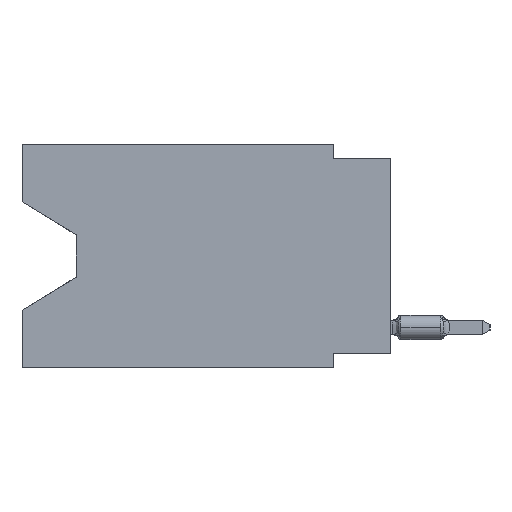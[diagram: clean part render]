
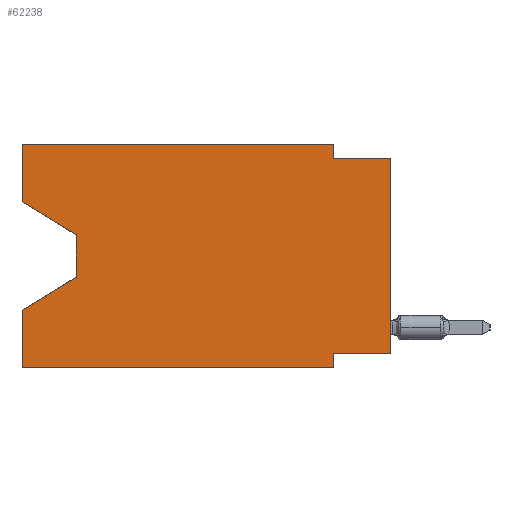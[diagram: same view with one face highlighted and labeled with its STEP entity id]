
A CAD part, left-side view. The second image highlights one B-rep face of the part: STEP entity #62238.
In plain terms, the highlighted planar face has unit normal (-1, 0, 0).
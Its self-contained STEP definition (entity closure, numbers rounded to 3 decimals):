
#249 = DIRECTION ( 'NONE',  ( 0., -0.855, -0.519 ) ) ;
#946 = ORIENTED_EDGE ( 'NONE', *, *, #59350, .F. ) ;
#1407 = PLANE ( 'NONE',  #7633 ) ;
#1590 = LINE ( 'NONE', #39635, #60868 ) ;
#2728 = VERTEX_POINT ( 'NONE', #63224 ) ;
#3511 = DIRECTION ( 'NONE',  ( 0., 0., 1. ) ) ;
#5503 = LINE ( 'NONE', #48896, #59118 ) ;
#5581 = EDGE_CURVE ( 'NONE', #42750, #20444, #65869, .T. ) ;
#6295 = CARTESIAN_POINT ( 'NONE',  ( 0., 16.383, -2.546 ) ) ;
#7633 = AXIS2_PLACEMENT_3D ( 'NONE', #13825, #45502, #29827 ) ;
#7803 = CARTESIAN_POINT ( 'NONE',  ( 0., 16.383, 0. ) ) ;
#7955 = CARTESIAN_POINT ( 'NONE',  ( 0., 16.383, -9.906 ) ) ;
#8317 = EDGE_CURVE ( 'NONE', #41188, #2728, #55021, .T. ) ;
#9799 = EDGE_LOOP ( 'NONE', ( #11325, #43804, #39291, #16638, #15266, #60975, #36947, #10320, #946, #68223, #22908, #34133 ) ) ;
#10320 = ORIENTED_EDGE ( 'NONE', *, *, #64534, .T. ) ;
#10864 = LINE ( 'NONE', #22938, #62389 ) ;
#11325 = ORIENTED_EDGE ( 'NONE', *, *, #8317, .T. ) ;
#13005 = VERTEX_POINT ( 'NONE', #7955 ) ;
#13118 = FACE_OUTER_BOUND ( 'NONE', #9799, .T. ) ;
#13825 = CARTESIAN_POINT ( 'NONE',  ( 0., 16.383, 0. ) ) ;
#15266 = ORIENTED_EDGE ( 'NONE', *, *, #35008, .T. ) ;
#16268 = VERTEX_POINT ( 'NONE', #18613 ) ;
#16638 = ORIENTED_EDGE ( 'NONE', *, *, #67916, .F. ) ;
#17736 = CARTESIAN_POINT ( 'NONE',  ( 0., 0., -0.635 ) ) ;
#18571 = CARTESIAN_POINT ( 'NONE',  ( 0., 2.54, -9.906 ) ) ;
#18613 = CARTESIAN_POINT ( 'NONE',  ( 0., 16.383, -7.36 ) ) ;
#18658 = CARTESIAN_POINT ( 'NONE',  ( 0., 16.383, 0. ) ) ;
#18669 = CARTESIAN_POINT ( 'NONE',  ( 0., 2.54, 0. ) ) ;
#18926 = EDGE_CURVE ( 'NONE', #2728, #20175, #41097, .T. ) ;
#19148 = CARTESIAN_POINT ( 'NONE',  ( 0., 2.54, -0.635 ) ) ;
#19552 = CARTESIAN_POINT ( 'NONE',  ( 0., 2.54, -9.906 ) ) ;
#19811 = CARTESIAN_POINT ( 'NONE',  ( 0., 13.97, -5.893 ) ) ;
#20015 = VECTOR ( 'NONE', #60515, 1000. ) ;
#20175 = VERTEX_POINT ( 'NONE', #19811 ) ;
#20191 = CARTESIAN_POINT ( 'NONE',  ( 0., 2.54, 0. ) ) ;
#20444 = VERTEX_POINT ( 'NONE', #33662 ) ;
#22908 = ORIENTED_EDGE ( 'NONE', *, *, #42894, .F. ) ;
#22938 = CARTESIAN_POINT ( 'NONE',  ( 0., 0., 0. ) ) ;
#24057 = CARTESIAN_POINT ( 'NONE',  ( 0., 0., -0.635 ) ) ;
#25178 = LINE ( 'NONE', #20191, #45902 ) ;
#25745 = DIRECTION ( 'NONE',  ( 0., 0., -1. ) ) ;
#29827 = DIRECTION ( 'NONE',  ( 0., 0., -1. ) ) ;
#30064 = VECTOR ( 'NONE', #63453, 1000. ) ;
#33662 = CARTESIAN_POINT ( 'NONE',  ( 0., 2.54, -9.271 ) ) ;
#34133 = ORIENTED_EDGE ( 'NONE', *, *, #68953, .F. ) ;
#35008 = EDGE_CURVE ( 'NONE', #13005, #57825, #5503, .T. ) ;
#36947 = ORIENTED_EDGE ( 'NONE', *, *, #5581, .F. ) ;
#37166 = DIRECTION ( 'NONE',  ( 0., -1., 0. ) ) ;
#37662 = EDGE_CURVE ( 'NONE', #41083, #51309, #25178, .T. ) ;
#38133 = VERTEX_POINT ( 'NONE', #24057 ) ;
#39291 = ORIENTED_EDGE ( 'NONE', *, *, #58633, .T. ) ;
#39635 = CARTESIAN_POINT ( 'NONE',  ( 0., 16.383, 0. ) ) ;
#40279 = LINE ( 'NONE', #18571, #59414 ) ;
#41083 = VERTEX_POINT ( 'NONE', #18669 ) ;
#41097 = LINE ( 'NONE', #63117, #50175 ) ;
#41188 = VERTEX_POINT ( 'NONE', #69485 ) ;
#42750 = VERTEX_POINT ( 'NONE', #57339 ) ;
#42894 = EDGE_CURVE ( 'NONE', #54156, #41083, #55663, .T. ) ;
#43804 = ORIENTED_EDGE ( 'NONE', *, *, #18926, .T. ) ;
#44990 = DIRECTION ( 'NONE',  ( 0., 0., 1. ) ) ;
#45502 = DIRECTION ( 'NONE',  ( 1., 0., 0. ) ) ;
#45852 = DIRECTION ( 'NONE',  ( 0., 0., -1. ) ) ;
#45902 = VECTOR ( 'NONE', #45852, 1000. ) ;
#46418 = CARTESIAN_POINT ( 'NONE',  ( 0., 13.97, -5.893 ) ) ;
#47455 = LINE ( 'NONE', #46418, #30064 ) ;
#47917 = EDGE_CURVE ( 'NONE', #20444, #57825, #40279, .T. ) ;
#48896 = CARTESIAN_POINT ( 'NONE',  ( 0., 16.383, -9.906 ) ) ;
#49879 = CARTESIAN_POINT ( 'NONE',  ( 0., 0., -9.271 ) ) ;
#50175 = VECTOR ( 'NONE', #25745, 1000. ) ;
#51302 = DIRECTION ( 'NONE',  ( 0., 0., -1. ) ) ;
#51309 = VERTEX_POINT ( 'NONE', #19148 ) ;
#54156 = VERTEX_POINT ( 'NONE', #68386 ) ;
#55021 = LINE ( 'NONE', #6295, #55649 ) ;
#55376 = VECTOR ( 'NONE', #3511, 1000. ) ;
#55649 = VECTOR ( 'NONE', #249, 1000. ) ;
#55663 = LINE ( 'NONE', #18658, #64528 ) ;
#56511 = LINE ( 'NONE', #7803, #55376 ) ;
#56705 = DIRECTION ( 'NONE',  ( 0., -1., 0. ) ) ;
#57339 = CARTESIAN_POINT ( 'NONE',  ( 0., 0., -9.271 ) ) ;
#57825 = VERTEX_POINT ( 'NONE', #19552 ) ;
#58633 = EDGE_CURVE ( 'NONE', #20175, #16268, #47455, .T. ) ;
#59118 = VECTOR ( 'NONE', #37166, 1000. ) ;
#59350 = EDGE_CURVE ( 'NONE', #51309, #38133, #66481, .T. ) ;
#59414 = VECTOR ( 'NONE', #51302, 1000. ) ;
#60275 = DIRECTION ( 'NONE',  ( 0., 0., 1. ) ) ;
#60515 = DIRECTION ( 'NONE',  ( 0., 1., 0. ) ) ;
#60868 = VECTOR ( 'NONE', #44990, 1000. ) ;
#60975 = ORIENTED_EDGE ( 'NONE', *, *, #47917, .F. ) ;
#61112 = DIRECTION ( 'NONE',  ( 0., -1., 0. ) ) ;
#62238 = ADVANCED_FACE ( 'NONE', ( #13118 ), #1407, .F. ) ;
#62389 = VECTOR ( 'NONE', #60275, 1000. ) ;
#63117 = CARTESIAN_POINT ( 'NONE',  ( 0., 13.97, -4.013 ) ) ;
#63224 = CARTESIAN_POINT ( 'NONE',  ( 0., 13.97, -4.013 ) ) ;
#63453 = DIRECTION ( 'NONE',  ( 0., 0.855, -0.519 ) ) ;
#64181 = VECTOR ( 'NONE', #61112, 1000. ) ;
#64528 = VECTOR ( 'NONE', #56705, 1000. ) ;
#64534 = EDGE_CURVE ( 'NONE', #42750, #38133, #10864, .T. ) ;
#65869 = LINE ( 'NONE', #49879, #20015 ) ;
#66481 = LINE ( 'NONE', #17736, #64181 ) ;
#67916 = EDGE_CURVE ( 'NONE', #13005, #16268, #1590, .T. ) ;
#68223 = ORIENTED_EDGE ( 'NONE', *, *, #37662, .F. ) ;
#68386 = CARTESIAN_POINT ( 'NONE',  ( 0., 16.383, 0. ) ) ;
#68953 = EDGE_CURVE ( 'NONE', #41188, #54156, #56511, .T. ) ;
#69485 = CARTESIAN_POINT ( 'NONE',  ( 0., 16.383, -2.546 ) ) ;
